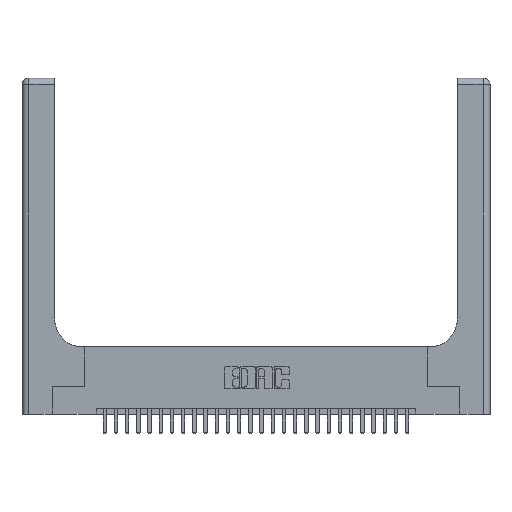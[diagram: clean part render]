
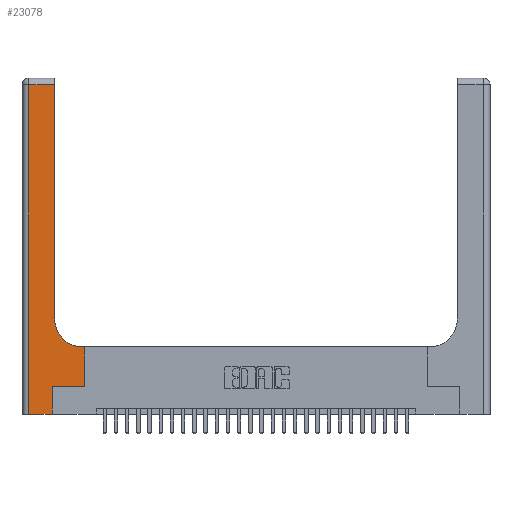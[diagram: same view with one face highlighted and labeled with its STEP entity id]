
A CAD part, top view. The second image highlights one B-rep face of the part: STEP entity #23078.
In plain terms, the highlighted planar face has unit normal (0, 0, 1).
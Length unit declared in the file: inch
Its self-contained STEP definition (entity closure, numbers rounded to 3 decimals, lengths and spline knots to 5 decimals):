
#1123 = EDGE_CURVE ( 'NONE', #14072, #27372, #6848, .T. ) ;
#2152 = CARTESIAN_POINT ( 'NONE',  ( 0.269, 0.25, 0.37 ) ) ;
#2178 = VERTEX_POINT ( 'NONE', #16664 ) ;
#2305 = LINE ( 'NONE', #8202, #25549 ) ;
#3261 = CARTESIAN_POINT ( 'NONE',  ( 0.5585, 0.25, 0.37 ) ) ;
#3466 = DIRECTION ( 'NONE',  ( 0., 1., 0. ) ) ;
#3862 = ORIENTED_EDGE ( 'NONE', *, *, #4681, .T. ) ;
#3897 = AXIS2_PLACEMENT_3D ( 'NONE', #6567, #28887, #15640 ) ;
#4542 = ORIENTED_EDGE ( 'NONE', *, *, #1123, .T. ) ;
#4681 = EDGE_CURVE ( 'NONE', #5667, #2178, #2305, .T. ) ;
#5315 = DIRECTION ( 'NONE',  ( 0., 0., -1. ) ) ;
#5422 = LINE ( 'NONE', #2152, #28481 ) ;
#5500 = ORIENTED_EDGE ( 'NONE', *, *, #7564, .T. ) ;
#5667 = VERTEX_POINT ( 'NONE', #16061 ) ;
#6567 = CARTESIAN_POINT ( 'NONE',  ( 0., 3., 0.37 ) ) ;
#6848 = LINE ( 'NONE', #3261, #28478 ) ;
#7058 = VECTOR ( 'NONE', #16790, 39.37008 ) ;
#7564 = EDGE_CURVE ( 'NONE', #18533, #17288, #12160, .T. ) ;
#7914 = VERTEX_POINT ( 'NONE', #23967 ) ;
#8202 = CARTESIAN_POINT ( 'NONE',  ( 0., 0., 0.37 ) ) ;
#8840 = ORIENTED_EDGE ( 'NONE', *, *, #28656, .T. ) ;
#11150 = ORIENTED_EDGE ( 'NONE', *, *, #18825, .T. ) ;
#11622 = CARTESIAN_POINT ( 'NONE',  ( 0.06, 3., 0.37 ) ) ;
#12160 = LINE ( 'NONE', #16250, #29146 ) ;
#12450 = DIRECTION ( 'NONE',  ( -1., 0., 0. ) ) ;
#13364 = CARTESIAN_POINT ( 'NONE',  ( 0.2915, 0.85, 0.37 ) ) ;
#14072 = VERTEX_POINT ( 'NONE', #23674 ) ;
#14146 = LINE ( 'NONE', #23538, #19365 ) ;
#14425 = CARTESIAN_POINT ( 'NONE',  ( 0.2915, 0.6, 0.37 ) ) ;
#15640 = DIRECTION ( 'NONE',  ( -1., 0., 0. ) ) ;
#16061 = CARTESIAN_POINT ( 'NONE',  ( 0.06, 0., 0.37 ) ) ;
#16250 = CARTESIAN_POINT ( 'NONE',  ( 0.2915, 3., 0.37 ) ) ;
#16664 = CARTESIAN_POINT ( 'NONE',  ( 0.269, 0., 0.37 ) ) ;
#16790 = DIRECTION ( 'NONE',  ( -1., 0., 0. ) ) ;
#17288 = VERTEX_POINT ( 'NONE', #19930 ) ;
#17456 = CIRCLE ( 'NONE', #28810, 0.25 ) ;
#18447 = DIRECTION ( 'NONE',  ( 0., 1., 0. ) ) ;
#18533 = VERTEX_POINT ( 'NONE', #13364 ) ;
#18775 = CARTESIAN_POINT ( 'NONE',  ( 0.5415, 0.85, 0.37 ) ) ;
#18825 = EDGE_CURVE ( 'NONE', #7914, #18533, #17456, .T. ) ;
#18978 = LINE ( 'NONE', #14425, #7058 ) ;
#19329 = CARTESIAN_POINT ( 'NONE',  ( 0.06, 2.94, 0.37 ) ) ;
#19365 = VECTOR ( 'NONE', #12450, 39.37008 ) ;
#19471 = VERTEX_POINT ( 'NONE', #19329 ) ;
#19688 = VECTOR ( 'NONE', #22164, 39.37008 ) ;
#19930 = CARTESIAN_POINT ( 'NONE',  ( 0.2915, 2.94, 0.37 ) ) ;
#20659 = EDGE_CURVE ( 'NONE', #19471, #5667, #24595, .T. ) ;
#21013 = DIRECTION ( 'NONE',  ( 1., 0., 0. ) ) ;
#21054 = VERTEX_POINT ( 'NONE', #24343 ) ;
#21863 = EDGE_CURVE ( 'NONE', #27372, #7914, #18978, .T. ) ;
#22164 = DIRECTION ( 'NONE',  ( 0., 1., 0. ) ) ;
#22477 = DIRECTION ( 'NONE',  ( 1., 0., 0. ) ) ;
#22491 = CARTESIAN_POINT ( 'NONE',  ( 0.5585, 0.6, 0.37 ) ) ;
#22562 = ORIENTED_EDGE ( 'NONE', *, *, #23979, .T. ) ;
#22954 = EDGE_LOOP ( 'NONE', ( #5500, #22562, #26855, #3862, #28771, #8840, #4542, #28930, #11150 ) ) ;
#23078 = ADVANCED_FACE ( 'NONE', ( #24169 ), #28792, .F. ) ;
#23538 = CARTESIAN_POINT ( 'NONE',  ( 0., 2.94, 0.37 ) ) ;
#23674 = CARTESIAN_POINT ( 'NONE',  ( 0.5585, 0.25, 0.37 ) ) ;
#23835 = DIRECTION ( 'NONE',  ( 1., 0., 0. ) ) ;
#23967 = CARTESIAN_POINT ( 'NONE',  ( 0.5415, 0.6, 0.37 ) ) ;
#23979 = EDGE_CURVE ( 'NONE', #17288, #19471, #14146, .T. ) ;
#24169 = FACE_OUTER_BOUND ( 'NONE', #22954, .T. ) ;
#24237 = EDGE_CURVE ( 'NONE', #2178, #21054, #24883, .T. ) ;
#24343 = CARTESIAN_POINT ( 'NONE',  ( 0.269, 0.25, 0.37 ) ) ;
#24595 = LINE ( 'NONE', #11622, #25303 ) ;
#24883 = LINE ( 'NONE', #28816, #19688 ) ;
#25045 = DIRECTION ( 'NONE',  ( 0., -1., 0. ) ) ;
#25303 = VECTOR ( 'NONE', #25045, 39.37008 ) ;
#25549 = VECTOR ( 'NONE', #23835, 39.37008 ) ;
#26855 = ORIENTED_EDGE ( 'NONE', *, *, #20659, .T. ) ;
#27372 = VERTEX_POINT ( 'NONE', #22491 ) ;
#28478 = VECTOR ( 'NONE', #3466, 39.37008 ) ;
#28481 = VECTOR ( 'NONE', #22477, 39.37008 ) ;
#28656 = EDGE_CURVE ( 'NONE', #21054, #14072, #5422, .T. ) ;
#28771 = ORIENTED_EDGE ( 'NONE', *, *, #24237, .T. ) ;
#28792 = PLANE ( 'NONE',  #3897 ) ;
#28810 = AXIS2_PLACEMENT_3D ( 'NONE', #18775, #5315, #21013 ) ;
#28816 = CARTESIAN_POINT ( 'NONE',  ( 0.269, 0., 0.37 ) ) ;
#28887 = DIRECTION ( 'NONE',  ( 0., 0., -1. ) ) ;
#28930 = ORIENTED_EDGE ( 'NONE', *, *, #21863, .T. ) ;
#29146 = VECTOR ( 'NONE', #18447, 39.37008 ) ;
